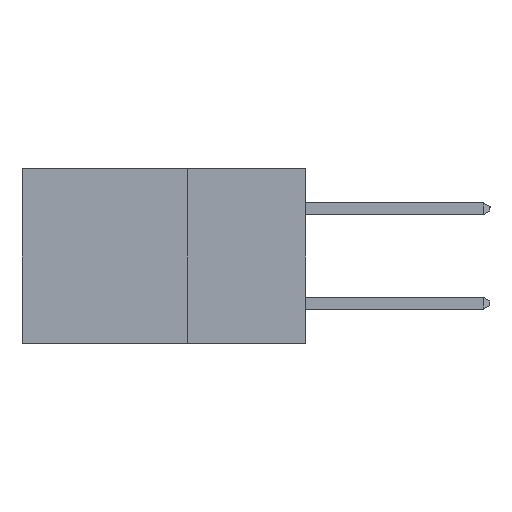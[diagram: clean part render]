
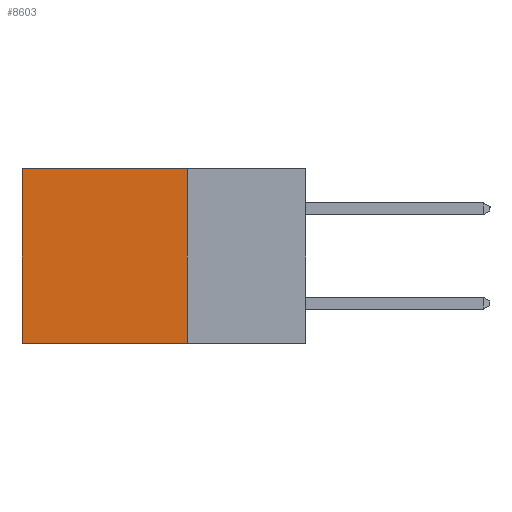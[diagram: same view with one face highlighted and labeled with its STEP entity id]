
A CAD part, left-side view. The second image highlights one B-rep face of the part: STEP entity #8603.
In plain terms, the highlighted planar face has unit normal (-1, 0, 0).
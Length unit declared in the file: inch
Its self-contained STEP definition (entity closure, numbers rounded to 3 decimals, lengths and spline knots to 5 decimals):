
#577 = DIRECTION ( 'NONE',  ( 0., 1., 0. ) ) ;
#627 = ORIENTED_EDGE ( 'NONE', *, *, #9138, .F. ) ;
#682 = CARTESIAN_POINT ( 'NONE',  ( 0.2615, 0.6, 0. ) ) ;
#736 = ORIENTED_EDGE ( 'NONE', *, *, #9260, .T. ) ;
#844 = VECTOR ( 'NONE', #7072, 39.37008 ) ;
#968 = DIRECTION ( 'NONE',  ( 0., 0., -1. ) ) ;
#1070 = LINE ( 'NONE', #7742, #6944 ) ;
#1737 = LINE ( 'NONE', #10715, #6529 ) ;
#2284 = EDGE_CURVE ( 'NONE', #4038, #2564, #7018, .T. ) ;
#2564 = VERTEX_POINT ( 'NONE', #5150 ) ;
#3416 = EDGE_CURVE ( 'NONE', #9986, #3610, #1070, .T. ) ;
#3610 = VERTEX_POINT ( 'NONE', #682 ) ;
#3762 = CARTESIAN_POINT ( 'NONE',  ( 0.2615, 0.25, -0.37 ) ) ;
#4038 = VERTEX_POINT ( 'NONE', #9978 ) ;
#4268 = PLANE ( 'NONE',  #9301 ) ;
#4538 = EDGE_LOOP ( 'NONE', ( #736, #7999, #627, #9160 ) ) ;
#5150 = CARTESIAN_POINT ( 'NONE',  ( 0.2615, 0.6, -0.37 ) ) ;
#5240 = DIRECTION ( 'NONE',  ( 1., 0., 0. ) ) ;
#5618 = DIRECTION ( 'NONE',  ( 0., 0., -1. ) ) ;
#6192 = VECTOR ( 'NONE', #5618, 39.37008 ) ;
#6529 = VECTOR ( 'NONE', #6748, 39.37008 ) ;
#6547 = CARTESIAN_POINT ( 'NONE',  ( 0.2615, 0.25, 0. ) ) ;
#6748 = DIRECTION ( 'NONE',  ( 0., 0., -1. ) ) ;
#6944 = VECTOR ( 'NONE', #577, 39.37008 ) ;
#7018 = LINE ( 'NONE', #3762, #844 ) ;
#7072 = DIRECTION ( 'NONE',  ( 0., 1., 0. ) ) ;
#7742 = CARTESIAN_POINT ( 'NONE',  ( 0.2615, 0.25, 0. ) ) ;
#7999 = ORIENTED_EDGE ( 'NONE', *, *, #2284, .F. ) ;
#8057 = LINE ( 'NONE', #10564, #6192 ) ;
#8603 = ADVANCED_FACE ( 'NONE', ( #9378 ), #4268, .F. ) ;
#9138 = EDGE_CURVE ( 'NONE', #9986, #4038, #8057, .T. ) ;
#9160 = ORIENTED_EDGE ( 'NONE', *, *, #3416, .T. ) ;
#9260 = EDGE_CURVE ( 'NONE', #3610, #2564, #1737, .T. ) ;
#9301 = AXIS2_PLACEMENT_3D ( 'NONE', #10084, #5240, #968 ) ;
#9378 = FACE_OUTER_BOUND ( 'NONE', #4538, .T. ) ;
#9978 = CARTESIAN_POINT ( 'NONE',  ( 0.2615, 0.25, -0.37 ) ) ;
#9986 = VERTEX_POINT ( 'NONE', #6547 ) ;
#10084 = CARTESIAN_POINT ( 'NONE',  ( 0.2615, 0.25, -0.37 ) ) ;
#10564 = CARTESIAN_POINT ( 'NONE',  ( 0.2615, 0.25, -0.37 ) ) ;
#10715 = CARTESIAN_POINT ( 'NONE',  ( 0.2615, 0.6, -0.37 ) ) ;
